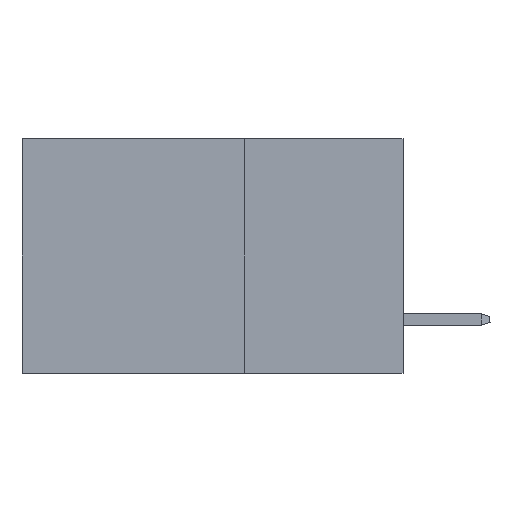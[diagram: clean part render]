
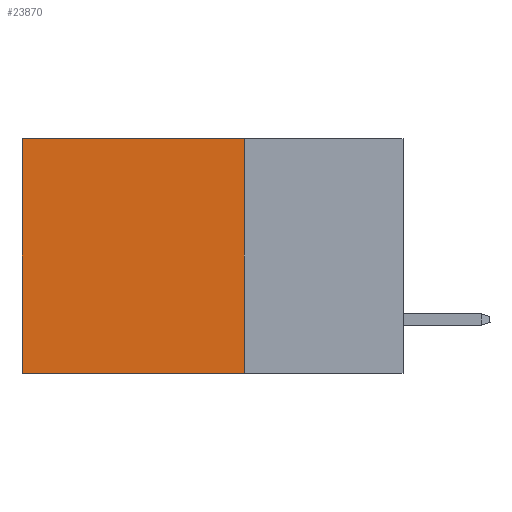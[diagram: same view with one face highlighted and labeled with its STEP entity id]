
A CAD part, left-side view. The second image highlights one B-rep face of the part: STEP entity #23870.
In plain terms, the highlighted planar face has unit normal (-1, 0, 0).
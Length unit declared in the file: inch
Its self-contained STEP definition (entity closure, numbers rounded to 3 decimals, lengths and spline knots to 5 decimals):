
#839 = CARTESIAN_POINT ( 'NONE',  ( 0.2875, 0.25, -0.37 ) ) ;
#2806 = FACE_OUTER_BOUND ( 'NONE', #17214, .T. ) ;
#2935 = CARTESIAN_POINT ( 'NONE',  ( 0.2875, 0.25, 0. ) ) ;
#4300 = DIRECTION ( 'NONE',  ( 0., 0., -1. ) ) ;
#5454 = VECTOR ( 'NONE', #4300, 39.37008 ) ;
#5617 = DIRECTION ( 'NONE',  ( 0., 1., 0. ) ) ;
#6055 = CARTESIAN_POINT ( 'NONE',  ( 0.2875, 0.25, 0. ) ) ;
#6914 = EDGE_CURVE ( 'NONE', #18672, #16058, #18975, .T. ) ;
#8045 = EDGE_CURVE ( 'NONE', #28994, #16058, #13638, .T. ) ;
#10680 = ORIENTED_EDGE ( 'NONE', *, *, #28107, .T. ) ;
#12383 = VECTOR ( 'NONE', #23615, 39.37008 ) ;
#13638 = LINE ( 'NONE', #22664, #5454 ) ;
#13896 = VERTEX_POINT ( 'NONE', #25386 ) ;
#14195 = DIRECTION ( 'NONE',  ( 0., 0., -1. ) ) ;
#15076 = DIRECTION ( 'NONE',  ( 0., 1., 0. ) ) ;
#16058 = VERTEX_POINT ( 'NONE', #17406 ) ;
#16820 = LINE ( 'NONE', #25670, #12383 ) ;
#17019 = CARTESIAN_POINT ( 'NONE',  ( 0.2875, 0.25, -0.37 ) ) ;
#17155 = LINE ( 'NONE', #6055, #23899 ) ;
#17214 = EDGE_LOOP ( 'NONE', ( #27353, #28118, #23088, #10680 ) ) ;
#17389 = CARTESIAN_POINT ( 'NONE',  ( 0.2875, 0.6, 0. ) ) ;
#17406 = CARTESIAN_POINT ( 'NONE',  ( 0.2875, 0.6, -0.37 ) ) ;
#18672 = VERTEX_POINT ( 'NONE', #839 ) ;
#18975 = LINE ( 'NONE', #17019, #20054 ) ;
#20054 = VECTOR ( 'NONE', #5617, 39.37008 ) ;
#20542 = DIRECTION ( 'NONE',  ( 1., 0., 0. ) ) ;
#21712 = EDGE_CURVE ( 'NONE', #13896, #18672, #16820, .T. ) ;
#22664 = CARTESIAN_POINT ( 'NONE',  ( 0.2875, 0.6, 0. ) ) ;
#23088 = ORIENTED_EDGE ( 'NONE', *, *, #21712, .F. ) ;
#23196 = PLANE ( 'NONE',  #27967 ) ;
#23615 = DIRECTION ( 'NONE',  ( 0., 0., -1. ) ) ;
#23870 = ADVANCED_FACE ( 'NONE', ( #2806 ), #23196, .F. ) ;
#23899 = VECTOR ( 'NONE', #15076, 39.37008 ) ;
#25386 = CARTESIAN_POINT ( 'NONE',  ( 0.2875, 0.25, 0. ) ) ;
#25670 = CARTESIAN_POINT ( 'NONE',  ( 0.2875, 0.25, 0. ) ) ;
#27353 = ORIENTED_EDGE ( 'NONE', *, *, #8045, .T. ) ;
#27967 = AXIS2_PLACEMENT_3D ( 'NONE', #2935, #20542, #14195 ) ;
#28107 = EDGE_CURVE ( 'NONE', #13896, #28994, #17155, .T. ) ;
#28118 = ORIENTED_EDGE ( 'NONE', *, *, #6914, .F. ) ;
#28994 = VERTEX_POINT ( 'NONE', #17389 ) ;
